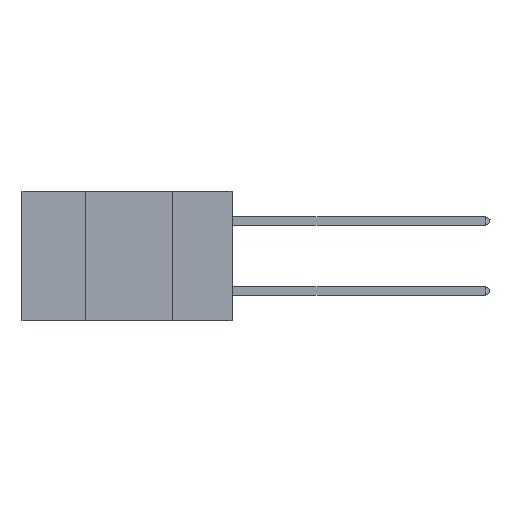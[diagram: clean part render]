
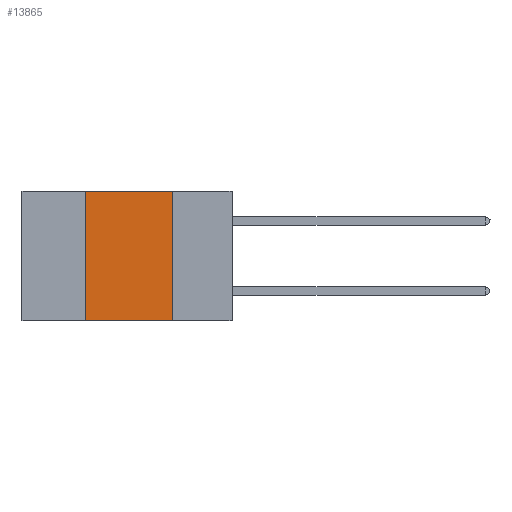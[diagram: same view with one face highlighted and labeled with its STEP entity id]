
A CAD part, left-side view. The second image highlights one B-rep face of the part: STEP entity #13865.
In plain terms, the highlighted planar face has unit normal (-1, 0, 0).
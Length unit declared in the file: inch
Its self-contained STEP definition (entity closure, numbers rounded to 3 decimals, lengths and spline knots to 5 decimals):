
#1560 = EDGE_LOOP ( 'NONE', ( #10948, #22398, #24323, #18504 ) ) ;
#1804 = VERTEX_POINT ( 'NONE', #22089 ) ;
#2545 = CARTESIAN_POINT ( 'NONE',  ( 0., 0.6, 0. ) ) ;
#2570 = VERTEX_POINT ( 'NONE', #11708 ) ;
#4704 = DIRECTION ( 'NONE',  ( 0., -1., 0. ) ) ;
#6020 = CARTESIAN_POINT ( 'NONE',  ( 0., 0.17, -0.37 ) ) ;
#7583 = VECTOR ( 'NONE', #8405, 39.37008 ) ;
#8405 = DIRECTION ( 'NONE',  ( 0., 0., 1. ) ) ;
#9177 = EDGE_CURVE ( 'NONE', #1804, #2570, #16226, .T. ) ;
#9413 = CARTESIAN_POINT ( 'NONE',  ( 0., 0.6, 0. ) ) ;
#10735 = LINE ( 'NONE', #12874, #16339 ) ;
#10948 = ORIENTED_EDGE ( 'NONE', *, *, #28438, .F. ) ;
#11708 = CARTESIAN_POINT ( 'NONE',  ( 0., 0.17, 0. ) ) ;
#12874 = CARTESIAN_POINT ( 'NONE',  ( 0., 0.6, -0.37 ) ) ;
#13234 = VERTEX_POINT ( 'NONE', #26982 ) ;
#13833 = VECTOR ( 'NONE', #18916, 39.37008 ) ;
#13845 = DIRECTION ( 'NONE',  ( 0., -1., 0. ) ) ;
#13865 = ADVANCED_FACE ( 'NONE', ( #21760 ), #27300, .F. ) ;
#15169 = CARTESIAN_POINT ( 'NONE',  ( 0., 0.42, 0. ) ) ;
#16226 = LINE ( 'NONE', #2545, #25705 ) ;
#16339 = VECTOR ( 'NONE', #4704, 39.37008 ) ;
#18504 = ORIENTED_EDGE ( 'NONE', *, *, #22933, .T. ) ;
#18652 = DIRECTION ( 'NONE',  ( 1., 0., 0. ) ) ;
#18916 = DIRECTION ( 'NONE',  ( 0., 0., -1. ) ) ;
#20391 = VERTEX_POINT ( 'NONE', #6020 ) ;
#21760 = FACE_OUTER_BOUND ( 'NONE', #1560, .T. ) ;
#21829 = AXIS2_PLACEMENT_3D ( 'NONE', #9413, #18652, #23171 ) ;
#22089 = CARTESIAN_POINT ( 'NONE',  ( 0., 0.42, 0. ) ) ;
#22256 = EDGE_CURVE ( 'NONE', #13234, #1804, #27983, .T. ) ;
#22398 = ORIENTED_EDGE ( 'NONE', *, *, #9177, .F. ) ;
#22933 = EDGE_CURVE ( 'NONE', #13234, #20391, #10735, .T. ) ;
#23171 = DIRECTION ( 'NONE',  ( 0., 0., -1. ) ) ;
#24323 = ORIENTED_EDGE ( 'NONE', *, *, #22256, .F. ) ;
#25705 = VECTOR ( 'NONE', #13845, 39.37008 ) ;
#26521 = LINE ( 'NONE', #28028, #13833 ) ;
#26982 = CARTESIAN_POINT ( 'NONE',  ( 0., 0.42, -0.37 ) ) ;
#27300 = PLANE ( 'NONE',  #21829 ) ;
#27983 = LINE ( 'NONE', #15169, #7583 ) ;
#28028 = CARTESIAN_POINT ( 'NONE',  ( 0., 0.17, 0. ) ) ;
#28438 = EDGE_CURVE ( 'NONE', #2570, #20391, #26521, .T. ) ;
